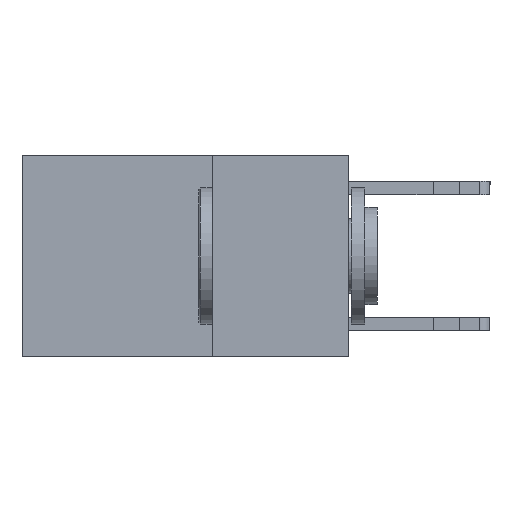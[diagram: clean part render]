
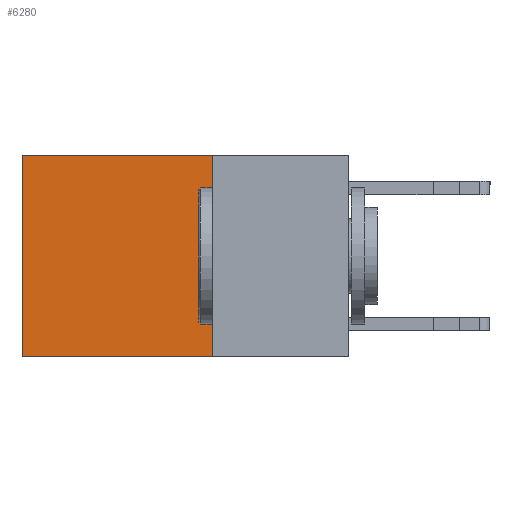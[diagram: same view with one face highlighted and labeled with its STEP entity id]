
A CAD part, left-side view. The second image highlights one B-rep face of the part: STEP entity #6280.
In plain terms, the highlighted planar face has unit normal (-1, 0, 0).
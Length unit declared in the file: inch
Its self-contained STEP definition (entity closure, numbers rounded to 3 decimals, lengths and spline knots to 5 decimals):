
#636 = LINE ( 'NONE', #14451, #1140 ) ;
#716 = EDGE_CURVE ( 'NONE', #1144, #15090, #1943, .T. ) ;
#718 = EDGE_CURVE ( 'NONE', #11795, #8531, #636, .T. ) ;
#743 = PLANE ( 'NONE',  #17420 ) ;
#1140 = VECTOR ( 'NONE', #9030, 39.37008 ) ;
#1144 = VERTEX_POINT ( 'NONE', #15730 ) ;
#1943 = LINE ( 'NONE', #17497, #12321 ) ;
#3513 = DIRECTION ( 'NONE',  ( 0., 1., 0. ) ) ;
#3613 = DIRECTION ( 'NONE',  ( 0., 0., -1. ) ) ;
#3665 = CARTESIAN_POINT ( 'NONE',  ( 0.2625, 0.25, -0.37 ) ) ;
#4136 = VECTOR ( 'NONE', #3513, 39.37008 ) ;
#4206 = ORIENTED_EDGE ( 'NONE', *, *, #718, .F. ) ;
#4534 = DIRECTION ( 'NONE',  ( 0., 0., -1. ) ) ;
#5368 = CARTESIAN_POINT ( 'NONE',  ( 0.2625, 0.25, 0. ) ) ;
#6280 = ADVANCED_FACE ( 'NONE', ( #10866 ), #743, .F. ) ;
#8156 = LINE ( 'NONE', #9540, #12080 ) ;
#8531 = VERTEX_POINT ( 'NONE', #3665 ) ;
#9030 = DIRECTION ( 'NONE',  ( 0., 0., -1. ) ) ;
#9376 = CARTESIAN_POINT ( 'NONE',  ( 0.2625, 0.25, 0. ) ) ;
#9540 = CARTESIAN_POINT ( 'NONE',  ( 0.2625, 0.25, -0.37 ) ) ;
#9625 = ORIENTED_EDGE ( 'NONE', *, *, #15217, .T. ) ;
#10265 = ORIENTED_EDGE ( 'NONE', *, *, #15605, .F. ) ;
#10866 = FACE_OUTER_BOUND ( 'NONE', #16153, .T. ) ;
#11795 = VERTEX_POINT ( 'NONE', #9376 ) ;
#12080 = VECTOR ( 'NONE', #17988, 39.37008 ) ;
#12321 = VECTOR ( 'NONE', #4534, 39.37008 ) ;
#13279 = ORIENTED_EDGE ( 'NONE', *, *, #716, .T. ) ;
#13718 = LINE ( 'NONE', #5368, #4136 ) ;
#14451 = CARTESIAN_POINT ( 'NONE',  ( 0.2625, 0.25, 0. ) ) ;
#14733 = DIRECTION ( 'NONE',  ( 1., 0., 0. ) ) ;
#15090 = VERTEX_POINT ( 'NONE', #16112 ) ;
#15217 = EDGE_CURVE ( 'NONE', #11795, #1144, #13718, .T. ) ;
#15605 = EDGE_CURVE ( 'NONE', #8531, #15090, #8156, .T. ) ;
#15730 = CARTESIAN_POINT ( 'NONE',  ( 0.2625, 0.6, 0. ) ) ;
#16112 = CARTESIAN_POINT ( 'NONE',  ( 0.2625, 0.6, -0.37 ) ) ;
#16153 = EDGE_LOOP ( 'NONE', ( #13279, #10265, #4206, #9625 ) ) ;
#17420 = AXIS2_PLACEMENT_3D ( 'NONE', #17850, #14733, #3613 ) ;
#17497 = CARTESIAN_POINT ( 'NONE',  ( 0.2625, 0.6, 0. ) ) ;
#17850 = CARTESIAN_POINT ( 'NONE',  ( 0.2625, 0.25, 0. ) ) ;
#17988 = DIRECTION ( 'NONE',  ( 0., 1., 0. ) ) ;
